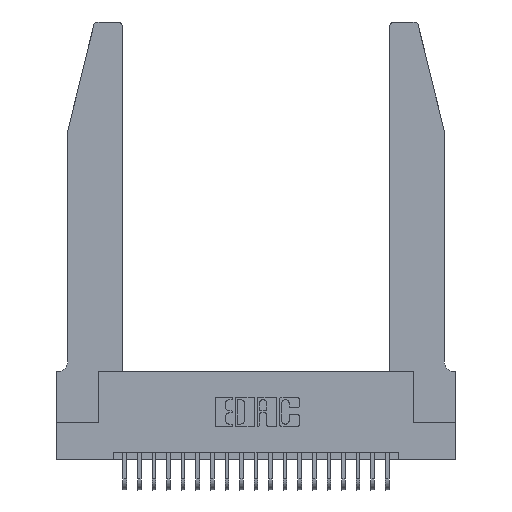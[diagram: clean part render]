
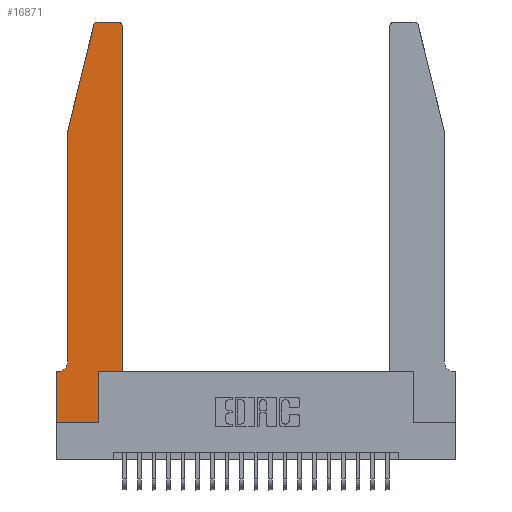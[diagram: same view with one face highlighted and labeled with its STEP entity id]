
A CAD part, top view. The second image highlights one B-rep face of the part: STEP entity #16871.
In plain terms, the highlighted planar face has unit normal (0, 0, 1).
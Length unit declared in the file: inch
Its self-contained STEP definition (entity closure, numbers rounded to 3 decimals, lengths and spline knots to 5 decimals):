
#512 = ORIENTED_EDGE ( 'NONE', *, *, #766, .T. ) ;
#630 = DIRECTION ( 'NONE',  ( 1., 0., 0. ) ) ;
#766 = EDGE_CURVE ( 'NONE', #6041, #20065, #5389, .T. ) ;
#863 = CIRCLE ( 'NONE', #3893, 0.03 ) ;
#895 = PLANE ( 'NONE',  #21996 ) ;
#905 = DIRECTION ( 'NONE',  ( 0., 0., 1. ) ) ;
#1161 = VECTOR ( 'NONE', #7998, 39.37008 ) ;
#1237 = CARTESIAN_POINT ( 'NONE',  ( 0.284, 2.72, 0.37 ) ) ;
#1499 = EDGE_CURVE ( 'NONE', #13709, #17806, #20675, .T. ) ;
#1537 = CARTESIAN_POINT ( 'NONE',  ( 0.0755, 2., 0.37 ) ) ;
#2065 = DIRECTION ( 'NONE',  ( 0., 1., 0. ) ) ;
#2701 = CARTESIAN_POINT ( 'NONE',  ( 0., 0.35, 0.37 ) ) ;
#2871 = EDGE_CURVE ( 'NONE', #18611, #14488, #6195, .T. ) ;
#3240 = FACE_OUTER_BOUND ( 'NONE', #17511, .T. ) ;
#3893 = AXIS2_PLACEMENT_3D ( 'NONE', #4900, #905, #12387 ) ;
#4193 = CARTESIAN_POINT ( 'NONE',  ( 0.284, 2.75, 0.37 ) ) ;
#4260 = ORIENTED_EDGE ( 'NONE', *, *, #14284, .T. ) ;
#4470 = CARTESIAN_POINT ( 'NONE',  ( 0.0755, 0.42, 0.37 ) ) ;
#4543 = CARTESIAN_POINT ( 'NONE',  ( 0., 0., 0.37 ) ) ;
#4661 = ORIENTED_EDGE ( 'NONE', *, *, #22849, .T. ) ;
#4900 = CARTESIAN_POINT ( 'NONE',  ( 0.4205, 2.72, 0.37 ) ) ;
#4915 = VECTOR ( 'NONE', #11119, 39.37008 ) ;
#5094 = LINE ( 'NONE', #13846, #13914 ) ;
#5389 = LINE ( 'NONE', #23191, #16035 ) ;
#5396 = ORIENTED_EDGE ( 'NONE', *, *, #9842, .T. ) ;
#5697 = EDGE_CURVE ( 'NONE', #17806, #6041, #18984, .T. ) ;
#5846 = CARTESIAN_POINT ( 'NONE',  ( 0.4205, 2.75, 0.37 ) ) ;
#6041 = VERTEX_POINT ( 'NONE', #8937 ) ;
#6195 = LINE ( 'NONE', #15488, #1161 ) ;
#6470 = CARTESIAN_POINT ( 'NONE',  ( 0.2865, 0., 0.37 ) ) ;
#6604 = DIRECTION ( 'NONE',  ( 1., 0., 0. ) ) ;
#7098 = EDGE_CURVE ( 'NONE', #21328, #23274, #5094, .T. ) ;
#7879 = LINE ( 'NONE', #1537, #4915 ) ;
#7998 = DIRECTION ( 'NONE',  ( 0., -1., 0. ) ) ;
#8187 = VECTOR ( 'NONE', #9983, 39.37008 ) ;
#8193 = DIRECTION ( 'NONE',  ( 0., -1., 0. ) ) ;
#8207 = ORIENTED_EDGE ( 'NONE', *, *, #20662, .T. ) ;
#8357 = CARTESIAN_POINT ( 'NONE',  ( 0.25487, 2.72718, 0.37 ) ) ;
#8656 = DIRECTION ( 'NONE',  ( -1., 0., 0. ) ) ;
#8744 = CARTESIAN_POINT ( 'NONE',  ( 0.4505, 0.35, 0.37 ) ) ;
#8937 = CARTESIAN_POINT ( 'NONE',  ( 0., 0., 0.37 ) ) ;
#8960 = DIRECTION ( 'NONE',  ( 1., 0., 0. ) ) ;
#9644 = LINE ( 'NONE', #19799, #8187 ) ;
#9842 = EDGE_CURVE ( 'NONE', #14488, #13709, #21108, .T. ) ;
#9983 = DIRECTION ( 'NONE',  ( 1., 0., 0. ) ) ;
#10149 = VECTOR ( 'NONE', #2065, 39.37008 ) ;
#10173 = CARTESIAN_POINT ( 'NONE',  ( 0.4505, 2.72, 0.37 ) ) ;
#10357 = DIRECTION ( 'NONE',  ( 0., 0., -1. ) ) ;
#11119 = DIRECTION ( 'NONE',  ( -0.239, -0.971, 0. ) ) ;
#11175 = CARTESIAN_POINT ( 'NONE',  ( 0.0755, 0.35, 0.37 ) ) ;
#11521 = EDGE_CURVE ( 'NONE', #14509, #18611, #7879, .T. ) ;
#12124 = DIRECTION ( 'NONE',  ( 0., 0., 1. ) ) ;
#12387 = DIRECTION ( 'NONE',  ( 1., 0., 0. ) ) ;
#12461 = ORIENTED_EDGE ( 'NONE', *, *, #2871, .T. ) ;
#12610 = CARTESIAN_POINT ( 'NONE',  ( 0., 0.35, 0.37 ) ) ;
#12750 = EDGE_CURVE ( 'NONE', #15637, #22336, #9644, .T. ) ;
#12816 = LINE ( 'NONE', #19300, #10149 ) ;
#13121 = ORIENTED_EDGE ( 'NONE', *, *, #20101, .T. ) ;
#13379 = VECTOR ( 'NONE', #8193, 39.37008 ) ;
#13709 = VERTEX_POINT ( 'NONE', #19252 ) ;
#13718 = AXIS2_PLACEMENT_3D ( 'NONE', #1237, #14546, #8960 ) ;
#13846 = CARTESIAN_POINT ( 'NONE',  ( 0.2605, 2.75, 0.37 ) ) ;
#13914 = VECTOR ( 'NONE', #23296, 39.37008 ) ;
#14284 = EDGE_CURVE ( 'NONE', #20065, #15637, #12816, .T. ) ;
#14488 = VERTEX_POINT ( 'NONE', #4470 ) ;
#14509 = VERTEX_POINT ( 'NONE', #8357 ) ;
#14546 = DIRECTION ( 'NONE',  ( 0., 0., 1. ) ) ;
#15306 = AXIS2_PLACEMENT_3D ( 'NONE', #19911, #10357, #8656 ) ;
#15488 = CARTESIAN_POINT ( 'NONE',  ( 0.0755, 2., 0.37 ) ) ;
#15503 = ORIENTED_EDGE ( 'NONE', *, *, #12750, .T. ) ;
#15637 = VERTEX_POINT ( 'NONE', #19505 ) ;
#15905 = DIRECTION ( 'NONE',  ( 0., 1., 0. ) ) ;
#16035 = VECTOR ( 'NONE', #6604, 39.37008 ) ;
#16499 = VECTOR ( 'NONE', #15905, 39.37008 ) ;
#16871 = ADVANCED_FACE ( 'NONE', ( #3240 ), #895, .T. ) ;
#17511 = EDGE_LOOP ( 'NONE', ( #18386, #4661, #21926, #12461, #5396, #22561, #21095, #512, #4260, #15503, #8207, #13121 ) ) ;
#17806 = VERTEX_POINT ( 'NONE', #12610 ) ;
#18386 = ORIENTED_EDGE ( 'NONE', *, *, #7098, .T. ) ;
#18539 = LINE ( 'NONE', #19436, #16499 ) ;
#18611 = VERTEX_POINT ( 'NONE', #20588 ) ;
#18984 = LINE ( 'NONE', #4543, #13379 ) ;
#19252 = CARTESIAN_POINT ( 'NONE',  ( 0.0055, 0.35, 0.37 ) ) ;
#19300 = CARTESIAN_POINT ( 'NONE',  ( 0.2865, 0.35, 0.37 ) ) ;
#19436 = CARTESIAN_POINT ( 'NONE',  ( 0.4505, 0.35, 0.37 ) ) ;
#19468 = VERTEX_POINT ( 'NONE', #10173 ) ;
#19505 = CARTESIAN_POINT ( 'NONE',  ( 0.2865, 0.35, 0.37 ) ) ;
#19799 = CARTESIAN_POINT ( 'NONE',  ( 0.4505, 0.35, 0.37 ) ) ;
#19911 = CARTESIAN_POINT ( 'NONE',  ( 0.0055, 0.42, 0.37 ) ) ;
#20065 = VERTEX_POINT ( 'NONE', #6470 ) ;
#20101 = EDGE_CURVE ( 'NONE', #19468, #21328, #863, .T. ) ;
#20459 = DIRECTION ( 'NONE',  ( -1., 0., 0. ) ) ;
#20588 = CARTESIAN_POINT ( 'NONE',  ( 0.0755, 2., 0.37 ) ) ;
#20662 = EDGE_CURVE ( 'NONE', #22336, #19468, #18539, .T. ) ;
#20675 = LINE ( 'NONE', #11175, #24216 ) ;
#21095 = ORIENTED_EDGE ( 'NONE', *, *, #5697, .T. ) ;
#21108 = CIRCLE ( 'NONE', #15306, 0.07 ) ;
#21328 = VERTEX_POINT ( 'NONE', #5846 ) ;
#21926 = ORIENTED_EDGE ( 'NONE', *, *, #11521, .T. ) ;
#21996 = AXIS2_PLACEMENT_3D ( 'NONE', #2701, #12124, #630 ) ;
#22261 = CIRCLE ( 'NONE', #13718, 0.03 ) ;
#22336 = VERTEX_POINT ( 'NONE', #8744 ) ;
#22561 = ORIENTED_EDGE ( 'NONE', *, *, #1499, .T. ) ;
#22849 = EDGE_CURVE ( 'NONE', #23274, #14509, #22261, .T. ) ;
#23191 = CARTESIAN_POINT ( 'NONE',  ( 0., 0., 0.37 ) ) ;
#23274 = VERTEX_POINT ( 'NONE', #4193 ) ;
#23296 = DIRECTION ( 'NONE',  ( -1., 0., 0. ) ) ;
#24216 = VECTOR ( 'NONE', #20459, 39.37008 ) ;
